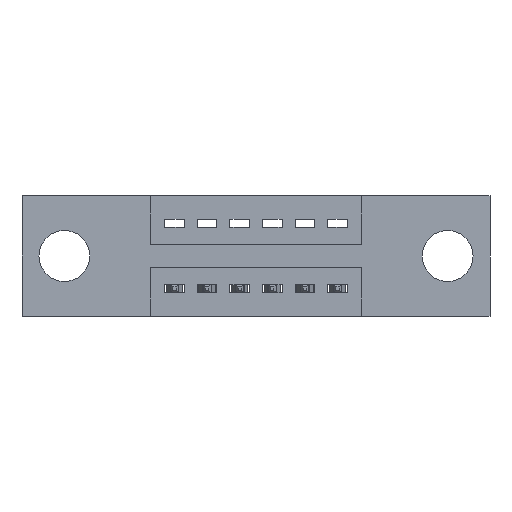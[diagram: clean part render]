
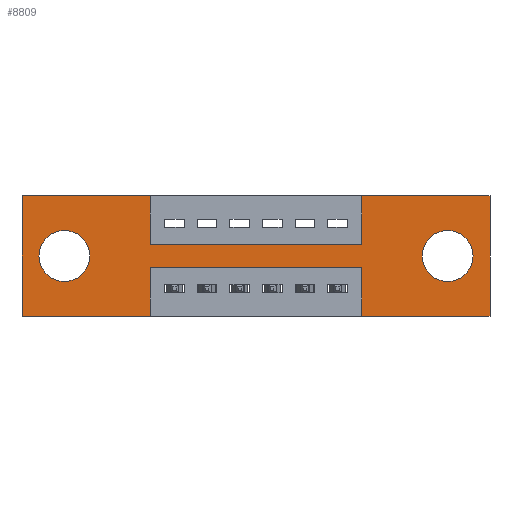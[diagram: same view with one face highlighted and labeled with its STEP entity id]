
A CAD part, front view. The second image highlights one B-rep face of the part: STEP entity #8809.
In plain terms, the highlighted planar face has unit normal (0, -1, 0).
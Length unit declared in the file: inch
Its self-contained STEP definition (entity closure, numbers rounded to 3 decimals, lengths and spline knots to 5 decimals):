
#2 = EDGE_CURVE ( 'NONE', #4861, #4478, #4213, .T. ) ;
#51 = CARTESIAN_POINT ( 'NONE',  ( 1.0425, 0., 0. ) ) ;
#114 = VECTOR ( 'NONE', #6732, 39.37008 ) ;
#126 = VERTEX_POINT ( 'NONE', #9281 ) ;
#150 = EDGE_CURVE ( 'NONE', #3994, #4626, #3070, .T. ) ;
#221 = CIRCLE ( 'NONE', #6923, 0.078 ) ;
#236 = VERTEX_POINT ( 'NONE', #5602 ) ;
#285 = CARTESIAN_POINT ( 'NONE',  ( 0.3925, 0., -0.15 ) ) ;
#510 = DIRECTION ( 'NONE',  ( 0., 0., -1. ) ) ;
#615 = CARTESIAN_POINT ( 'NONE',  ( 0., 0., 0. ) ) ;
#731 = CARTESIAN_POINT ( 'NONE',  ( 0.3925, 0., 0. ) ) ;
#772 = VERTEX_POINT ( 'NONE', #8280 ) ;
#825 = DIRECTION ( 'NONE',  ( 0., 1., 0. ) ) ;
#916 = DIRECTION ( 'NONE',  ( 0., 0., 1. ) ) ;
#926 = LINE ( 'NONE', #4102, #4345 ) ;
#948 = AXIS2_PLACEMENT_3D ( 'NONE', #4890, #2513, #6516 ) ;
#1019 = CARTESIAN_POINT ( 'NONE',  ( 0., 0., 0. ) ) ;
#1121 = EDGE_CURVE ( 'NONE', #9075, #4108, #5324, .T. ) ;
#1194 = DIRECTION ( 'NONE',  ( -1., 0., 0. ) ) ;
#1242 = PLANE ( 'NONE',  #2741 ) ;
#1342 = ORIENTED_EDGE ( 'NONE', *, *, #5969, .F. ) ;
#1359 = DIRECTION ( 'NONE',  ( 0., 0., -1. ) ) ;
#1481 = CARTESIAN_POINT ( 'NONE',  ( 0.13, 0., -0.185 ) ) ;
#1548 = CARTESIAN_POINT ( 'NONE',  ( 0., 0., 0. ) ) ;
#1572 = VECTOR ( 'NONE', #916, 39.37008 ) ;
#1629 = CARTESIAN_POINT ( 'NONE',  ( 1.305, 0., -0.107 ) ) ;
#1669 = DIRECTION ( 'NONE',  ( -1., 0., 0. ) ) ;
#1697 = VECTOR ( 'NONE', #1669, 39.37008 ) ;
#1717 = DIRECTION ( 'NONE',  ( 0., 0., -1. ) ) ;
#1725 = CARTESIAN_POINT ( 'NONE',  ( 1.305, 0., -0.263 ) ) ;
#1774 = CARTESIAN_POINT ( 'NONE',  ( 1.0425, 0., -0.37 ) ) ;
#1883 = LINE ( 'NONE', #615, #2577 ) ;
#1919 = VECTOR ( 'NONE', #7619, 39.37008 ) ;
#2171 = CARTESIAN_POINT ( 'NONE',  ( 1.435, 0., 0. ) ) ;
#2284 = LINE ( 'NONE', #3083, #1697 ) ;
#2377 = ORIENTED_EDGE ( 'NONE', *, *, #1121, .F. ) ;
#2394 = VERTEX_POINT ( 'NONE', #1725 ) ;
#2513 = DIRECTION ( 'NONE',  ( 0., 1., 0. ) ) ;
#2543 = VERTEX_POINT ( 'NONE', #4699 ) ;
#2577 = VECTOR ( 'NONE', #6570, 39.37008 ) ;
#2663 = CARTESIAN_POINT ( 'NONE',  ( 1.0425, 0., 0. ) ) ;
#2672 = DIRECTION ( 'NONE',  ( 0., 0., 1. ) ) ;
#2739 = CARTESIAN_POINT ( 'NONE',  ( 0.3925, 0., -0.37 ) ) ;
#2741 = AXIS2_PLACEMENT_3D ( 'NONE', #7024, #5578, #4089 ) ;
#2814 = EDGE_CURVE ( 'NONE', #4478, #3130, #8248, .T. ) ;
#2995 = ORIENTED_EDGE ( 'NONE', *, *, #2, .F. ) ;
#3070 = LINE ( 'NONE', #2739, #5685 ) ;
#3083 = CARTESIAN_POINT ( 'NONE',  ( 0., 0., -0.37 ) ) ;
#3130 = VERTEX_POINT ( 'NONE', #285 ) ;
#3151 = DIRECTION ( 'NONE',  ( 0., 1., 0. ) ) ;
#3198 = VECTOR ( 'NONE', #2672, 39.37008 ) ;
#3270 = CARTESIAN_POINT ( 'NONE',  ( 0.3925, 0., -0.15 ) ) ;
#3323 = CARTESIAN_POINT ( 'NONE',  ( 1.435, 0., -0.37 ) ) ;
#3398 = EDGE_CURVE ( 'NONE', #4804, #126, #8117, .T. ) ;
#3478 = FACE_BOUND ( 'NONE', #4359, .T. ) ;
#3689 = ORIENTED_EDGE ( 'NONE', *, *, #7417, .F. ) ;
#3723 = ORIENTED_EDGE ( 'NONE', *, *, #7477, .F. ) ;
#3748 = VECTOR ( 'NONE', #3812, 39.37008 ) ;
#3776 = LINE ( 'NONE', #2171, #6366 ) ;
#3779 = ORIENTED_EDGE ( 'NONE', *, *, #6495, .F. ) ;
#3812 = DIRECTION ( 'NONE',  ( -1., 0., 0. ) ) ;
#3987 = EDGE_CURVE ( 'NONE', #2394, #8642, #6523, .T. ) ;
#3994 = VERTEX_POINT ( 'NONE', #7463 ) ;
#4089 = DIRECTION ( 'NONE',  ( 0., 0., -1. ) ) ;
#4102 = CARTESIAN_POINT ( 'NONE',  ( 0.3925, 0., -0.22 ) ) ;
#4108 = VERTEX_POINT ( 'NONE', #2663 ) ;
#4213 = LINE ( 'NONE', #1019, #114 ) ;
#4345 = VECTOR ( 'NONE', #1194, 39.37008 ) ;
#4359 = EDGE_LOOP ( 'NONE', ( #5470, #8174 ) ) ;
#4478 = VERTEX_POINT ( 'NONE', #4818 ) ;
#4599 = ORIENTED_EDGE ( 'NONE', *, *, #6287, .F. ) ;
#4626 = VERTEX_POINT ( 'NONE', #8472 ) ;
#4673 = LINE ( 'NONE', #1774, #1572 ) ;
#4699 = CARTESIAN_POINT ( 'NONE',  ( 1.0425, 0., -0.37 ) ) ;
#4804 = VERTEX_POINT ( 'NONE', #7950 ) ;
#4818 = CARTESIAN_POINT ( 'NONE',  ( 0.3925, 0., 0. ) ) ;
#4861 = VERTEX_POINT ( 'NONE', #1548 ) ;
#4890 = CARTESIAN_POINT ( 'NONE',  ( 0.13, 0., -0.185 ) ) ;
#4901 = CARTESIAN_POINT ( 'NONE',  ( 0., 0., 0. ) ) ;
#4994 = VECTOR ( 'NONE', #6458, 39.37008 ) ;
#5191 = DIRECTION ( 'NONE',  ( 0., 0., -1. ) ) ;
#5278 = CARTESIAN_POINT ( 'NONE',  ( 1.0425, 0., -0.22 ) ) ;
#5324 = LINE ( 'NONE', #51, #4994 ) ;
#5470 = ORIENTED_EDGE ( 'NONE', *, *, #8922, .T. ) ;
#5537 = FACE_OUTER_BOUND ( 'NONE', #7398, .T. ) ;
#5578 = DIRECTION ( 'NONE',  ( 0., -1., 0. ) ) ;
#5602 = CARTESIAN_POINT ( 'NONE',  ( 0., 0., -0.37 ) ) ;
#5685 = VECTOR ( 'NONE', #510, 39.37008 ) ;
#5763 = CARTESIAN_POINT ( 'NONE',  ( 1.305, 0., -0.185 ) ) ;
#5969 = EDGE_CURVE ( 'NONE', #772, #7820, #3776, .T. ) ;
#5994 = VECTOR ( 'NONE', #1359, 39.37008 ) ;
#6123 = CARTESIAN_POINT ( 'NONE',  ( 0., 0., -0.37 ) ) ;
#6287 = EDGE_CURVE ( 'NONE', #7493, #3994, #926, .T. ) ;
#6363 = ORIENTED_EDGE ( 'NONE', *, *, #7530, .F. ) ;
#6366 = VECTOR ( 'NONE', #5191, 39.37008 ) ;
#6445 = DIRECTION ( 'NONE',  ( 0., 0., -1. ) ) ;
#6458 = DIRECTION ( 'NONE',  ( 0., 0., 1. ) ) ;
#6495 = EDGE_CURVE ( 'NONE', #236, #4861, #8970, .T. ) ;
#6516 = DIRECTION ( 'NONE',  ( 0., 0., 1. ) ) ;
#6523 = CIRCLE ( 'NONE', #6853, 0.078 ) ;
#6570 = DIRECTION ( 'NONE',  ( 1., 0., 0. ) ) ;
#6732 = DIRECTION ( 'NONE',  ( 1., 0., 0. ) ) ;
#6853 = AXIS2_PLACEMENT_3D ( 'NONE', #8903, #3151, #1717 ) ;
#6897 = EDGE_CURVE ( 'NONE', #126, #4804, #221, .T. ) ;
#6923 = AXIS2_PLACEMENT_3D ( 'NONE', #1481, #825, #7982 ) ;
#7024 = CARTESIAN_POINT ( 'NONE',  ( 0., 0., -0.37 ) ) ;
#7256 = ORIENTED_EDGE ( 'NONE', *, *, #2814, .F. ) ;
#7314 = FACE_BOUND ( 'NONE', #7421, .T. ) ;
#7334 = ORIENTED_EDGE ( 'NONE', *, *, #6897, .T. ) ;
#7398 = EDGE_LOOP ( 'NONE', ( #7943, #4599, #9084, #3723, #1342, #8205, #2377, #6363, #7256, #2995, #3779, #3689 ) ) ;
#7417 = EDGE_CURVE ( 'NONE', #4626, #236, #2284, .T. ) ;
#7421 = EDGE_LOOP ( 'NONE', ( #7334, #7686 ) ) ;
#7463 = CARTESIAN_POINT ( 'NONE',  ( 0.3925, 0., -0.22 ) ) ;
#7477 = EDGE_CURVE ( 'NONE', #7820, #2543, #7804, .T. ) ;
#7480 = EDGE_CURVE ( 'NONE', #2543, #7493, #4673, .T. ) ;
#7493 = VERTEX_POINT ( 'NONE', #5278 ) ;
#7530 = EDGE_CURVE ( 'NONE', #3130, #9075, #8154, .T. ) ;
#7619 = DIRECTION ( 'NONE',  ( 1., 0., 0. ) ) ;
#7658 = CIRCLE ( 'NONE', #9344, 0.078 ) ;
#7686 = ORIENTED_EDGE ( 'NONE', *, *, #3398, .T. ) ;
#7804 = LINE ( 'NONE', #6123, #3748 ) ;
#7820 = VERTEX_POINT ( 'NONE', #3323 ) ;
#7943 = ORIENTED_EDGE ( 'NONE', *, *, #150, .F. ) ;
#7950 = CARTESIAN_POINT ( 'NONE',  ( 0.13, 0., -0.263 ) ) ;
#7982 = DIRECTION ( 'NONE',  ( 0., 0., 1. ) ) ;
#8117 = CIRCLE ( 'NONE', #948, 0.078 ) ;
#8154 = LINE ( 'NONE', #3270, #1919 ) ;
#8174 = ORIENTED_EDGE ( 'NONE', *, *, #3987, .T. ) ;
#8205 = ORIENTED_EDGE ( 'NONE', *, *, #9185, .F. ) ;
#8248 = LINE ( 'NONE', #731, #5994 ) ;
#8280 = CARTESIAN_POINT ( 'NONE',  ( 1.435, 0., 0. ) ) ;
#8472 = CARTESIAN_POINT ( 'NONE',  ( 0.3925, 0., -0.37 ) ) ;
#8627 = DIRECTION ( 'NONE',  ( 0., 1., 0. ) ) ;
#8642 = VERTEX_POINT ( 'NONE', #1629 ) ;
#8809 = ADVANCED_FACE ( 'NONE', ( #3478, #7314, #5537 ), #1242, .T. ) ;
#8880 = CARTESIAN_POINT ( 'NONE',  ( 1.0425, 0., -0.15 ) ) ;
#8903 = CARTESIAN_POINT ( 'NONE',  ( 1.305, 0., -0.185 ) ) ;
#8922 = EDGE_CURVE ( 'NONE', #8642, #2394, #7658, .T. ) ;
#8970 = LINE ( 'NONE', #4901, #3198 ) ;
#9075 = VERTEX_POINT ( 'NONE', #8880 ) ;
#9084 = ORIENTED_EDGE ( 'NONE', *, *, #7480, .F. ) ;
#9185 = EDGE_CURVE ( 'NONE', #4108, #772, #1883, .T. ) ;
#9281 = CARTESIAN_POINT ( 'NONE',  ( 0.13, 0., -0.107 ) ) ;
#9344 = AXIS2_PLACEMENT_3D ( 'NONE', #5763, #8627, #6445 ) ;
